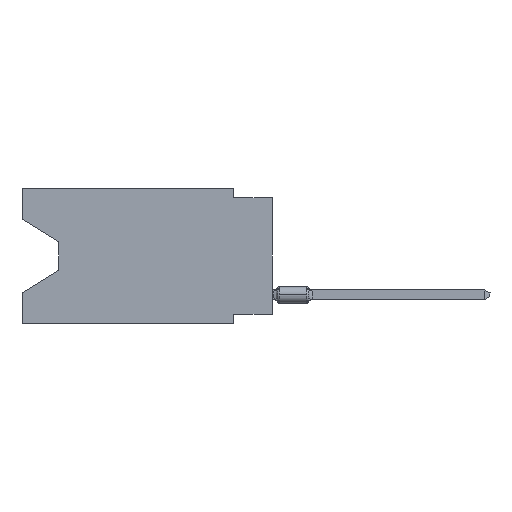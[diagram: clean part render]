
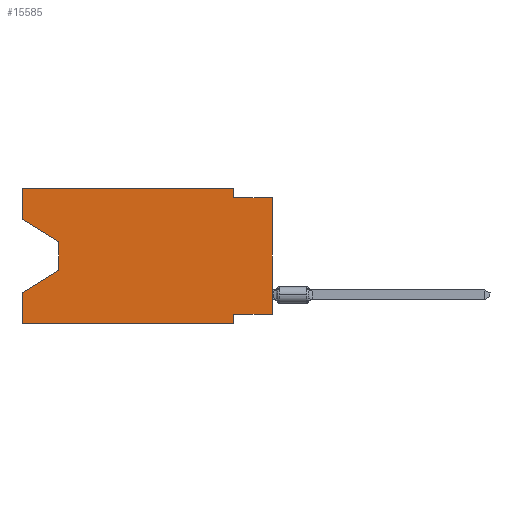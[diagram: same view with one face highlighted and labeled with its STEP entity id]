
A CAD part, left-side view. The second image highlights one B-rep face of the part: STEP entity #15585.
In plain terms, the highlighted planar face has unit normal (-1, 0, 0).
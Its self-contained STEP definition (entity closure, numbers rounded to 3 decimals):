
#1128 = DIRECTION ( 'NONE',  ( 0., 0., 1. ) ) ;
#1802 = CARTESIAN_POINT ( 'NONE',  ( 0., 16.383, -8.89 ) ) ;
#1861 = VERTEX_POINT ( 'NONE', #34820 ) ;
#2505 = VECTOR ( 'NONE', #82570, 1000. ) ;
#2726 = VECTOR ( 'NONE', #68338, 1000. ) ;
#2958 = CARTESIAN_POINT ( 'NONE',  ( 0., 16.383, 0. ) ) ;
#3372 = CARTESIAN_POINT ( 'NONE',  ( 0., 16.383, -8.89 ) ) ;
#3942 = CARTESIAN_POINT ( 'NONE',  ( 0., 2.54, 0. ) ) ;
#5047 = CARTESIAN_POINT ( 'NONE',  ( 0., 16.383, 0. ) ) ;
#5370 = VERTEX_POINT ( 'NONE', #55603 ) ;
#5539 = CARTESIAN_POINT ( 'NONE',  ( 0., 0., -0.635 ) ) ;
#5780 = DIRECTION ( 'NONE',  ( 0., 0., -1. ) ) ;
#6021 = CARTESIAN_POINT ( 'NONE',  ( 0., 0., -8.255 ) ) ;
#6452 = EDGE_CURVE ( 'NONE', #12702, #50448, #18759, .T. ) ;
#6673 = DIRECTION ( 'NONE',  ( 0., 0., -1. ) ) ;
#7310 = ORIENTED_EDGE ( 'NONE', *, *, #32930, .F. ) ;
#7333 = ORIENTED_EDGE ( 'NONE', *, *, #16170, .T. ) ;
#7348 = ORIENTED_EDGE ( 'NONE', *, *, #14038, .T. ) ;
#7464 = VECTOR ( 'NONE', #24768, 1000. ) ;
#8697 = DIRECTION ( 'NONE',  ( 0., 0., -1. ) ) ;
#10062 = LINE ( 'NONE', #67762, #51620 ) ;
#11160 = LINE ( 'NONE', #6021, #67222 ) ;
#12702 = VERTEX_POINT ( 'NONE', #81119 ) ;
#13268 = VERTEX_POINT ( 'NONE', #25853 ) ;
#14038 = EDGE_CURVE ( 'NONE', #26957, #50448, #60101, .T. ) ;
#14707 = EDGE_LOOP ( 'NONE', ( #25760, #77109, #7333, #81418, #79668, #43680, #27826, #7348, #64935, #75632, #79411, #7310 ) ) ;
#14765 = CARTESIAN_POINT ( 'NONE',  ( 0., 2.54, -8.255 ) ) ;
#15585 = ADVANCED_FACE ( 'NONE', ( #39522 ), #70295, .F. ) ;
#16170 = EDGE_CURVE ( 'NONE', #1861, #17158, #69257, .T. ) ;
#16369 = CARTESIAN_POINT ( 'NONE',  ( 0., 13.97, -3.505 ) ) ;
#16467 = DIRECTION ( 'NONE',  ( 0., 0., 1. ) ) ;
#16700 = DIRECTION ( 'NONE',  ( 0., 0.855, -0.519 ) ) ;
#16758 = LINE ( 'NONE', #3942, #2505 ) ;
#17158 = VERTEX_POINT ( 'NONE', #32619 ) ;
#18759 = LINE ( 'NONE', #5539, #7464 ) ;
#19028 = CARTESIAN_POINT ( 'NONE',  ( 0., 16.383, 0. ) ) ;
#20058 = EDGE_CURVE ( 'NONE', #13268, #50763, #10062, .T. ) ;
#24768 = DIRECTION ( 'NONE',  ( 0., -1., 0. ) ) ;
#25760 = ORIENTED_EDGE ( 'NONE', *, *, #20058, .T. ) ;
#25853 = CARTESIAN_POINT ( 'NONE',  ( 0., 16.383, -2.038 ) ) ;
#26176 = VECTOR ( 'NONE', #6673, 1000. ) ;
#26957 = VERTEX_POINT ( 'NONE', #68051 ) ;
#27252 = VECTOR ( 'NONE', #62216, 1000. ) ;
#27826 = ORIENTED_EDGE ( 'NONE', *, *, #76495, .F. ) ;
#28163 = EDGE_CURVE ( 'NONE', #5370, #12702, #16758, .T. ) ;
#30373 = CARTESIAN_POINT ( 'NONE',  ( 0., 13.97, -5.385 ) ) ;
#32009 = AXIS2_PLACEMENT_3D ( 'NONE', #19028, #77994, #5780 ) ;
#32619 = CARTESIAN_POINT ( 'NONE',  ( 0., 16.383, -6.852 ) ) ;
#32828 = VECTOR ( 'NONE', #55100, 1000. ) ;
#32930 = EDGE_CURVE ( 'NONE', #13268, #37264, #74592, .T. ) ;
#34820 = CARTESIAN_POINT ( 'NONE',  ( 0., 13.97, -5.385 ) ) ;
#37264 = VERTEX_POINT ( 'NONE', #5047 ) ;
#37424 = LINE ( 'NONE', #48991, #27252 ) ;
#37689 = EDGE_CURVE ( 'NONE', #69017, #17158, #37424, .T. ) ;
#37866 = LINE ( 'NONE', #78458, #26176 ) ;
#38903 = CARTESIAN_POINT ( 'NONE',  ( 0., 0., -0.635 ) ) ;
#39522 = FACE_OUTER_BOUND ( 'NONE', #14707, .T. ) ;
#40288 = VERTEX_POINT ( 'NONE', #83292 ) ;
#41281 = CARTESIAN_POINT ( 'NONE',  ( 0., 16.383, 0. ) ) ;
#42007 = LINE ( 'NONE', #16369, #72646 ) ;
#43680 = ORIENTED_EDGE ( 'NONE', *, *, #82241, .F. ) ;
#48963 = DIRECTION ( 'NONE',  ( 0., -0.855, -0.519 ) ) ;
#48991 = CARTESIAN_POINT ( 'NONE',  ( 0., 16.383, 0. ) ) ;
#50448 = VERTEX_POINT ( 'NONE', #38903 ) ;
#50763 = VERTEX_POINT ( 'NONE', #61906 ) ;
#51620 = VECTOR ( 'NONE', #48963, 1000. ) ;
#51913 = EDGE_CURVE ( 'NONE', #37264, #5370, #55511, .T. ) ;
#55100 = DIRECTION ( 'NONE',  ( 0., -1., 0. ) ) ;
#55511 = LINE ( 'NONE', #2958, #2726 ) ;
#55603 = CARTESIAN_POINT ( 'NONE',  ( 0., 2.54, 0. ) ) ;
#56355 = LINE ( 'NONE', #3372, #32828 ) ;
#56644 = VECTOR ( 'NONE', #16700, 1000. ) ;
#58232 = VERTEX_POINT ( 'NONE', #14765 ) ;
#59672 = CARTESIAN_POINT ( 'NONE',  ( 0., 0., 0. ) ) ;
#59949 = EDGE_CURVE ( 'NONE', #50763, #1861, #42007, .T. ) ;
#60101 = LINE ( 'NONE', #59672, #70184 ) ;
#60210 = VECTOR ( 'NONE', #16467, 1000. ) ;
#61906 = CARTESIAN_POINT ( 'NONE',  ( 0., 13.97, -3.505 ) ) ;
#62216 = DIRECTION ( 'NONE',  ( 0., 0., 1. ) ) ;
#64935 = ORIENTED_EDGE ( 'NONE', *, *, #6452, .F. ) ;
#67222 = VECTOR ( 'NONE', #83386, 1000. ) ;
#67762 = CARTESIAN_POINT ( 'NONE',  ( 0., 16.383, -2.038 ) ) ;
#68051 = CARTESIAN_POINT ( 'NONE',  ( 0., 0., -8.255 ) ) ;
#68338 = DIRECTION ( 'NONE',  ( 0., -1., 0. ) ) ;
#69017 = VERTEX_POINT ( 'NONE', #1802 ) ;
#69257 = LINE ( 'NONE', #30373, #56644 ) ;
#70184 = VECTOR ( 'NONE', #1128, 1000. ) ;
#70295 = PLANE ( 'NONE',  #32009 ) ;
#72646 = VECTOR ( 'NONE', #8697, 1000. ) ;
#74592 = LINE ( 'NONE', #41281, #60210 ) ;
#75632 = ORIENTED_EDGE ( 'NONE', *, *, #28163, .F. ) ;
#76495 = EDGE_CURVE ( 'NONE', #26957, #58232, #11160, .T. ) ;
#77109 = ORIENTED_EDGE ( 'NONE', *, *, #59949, .T. ) ;
#77994 = DIRECTION ( 'NONE',  ( 1., 0., 0. ) ) ;
#78458 = CARTESIAN_POINT ( 'NONE',  ( 0., 2.54, -8.89 ) ) ;
#79411 = ORIENTED_EDGE ( 'NONE', *, *, #51913, .F. ) ;
#79668 = ORIENTED_EDGE ( 'NONE', *, *, #80448, .T. ) ;
#80448 = EDGE_CURVE ( 'NONE', #69017, #40288, #56355, .T. ) ;
#81119 = CARTESIAN_POINT ( 'NONE',  ( 0., 2.54, -0.635 ) ) ;
#81418 = ORIENTED_EDGE ( 'NONE', *, *, #37689, .F. ) ;
#82241 = EDGE_CURVE ( 'NONE', #58232, #40288, #37866, .T. ) ;
#82570 = DIRECTION ( 'NONE',  ( 0., 0., -1. ) ) ;
#83292 = CARTESIAN_POINT ( 'NONE',  ( 0., 2.54, -8.89 ) ) ;
#83386 = DIRECTION ( 'NONE',  ( 0., 1., 0. ) ) ;
